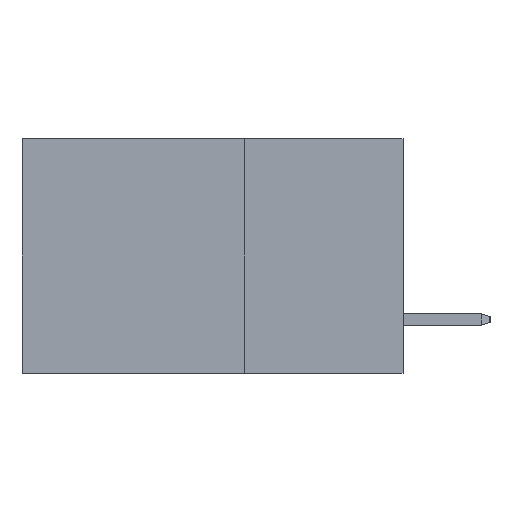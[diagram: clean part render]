
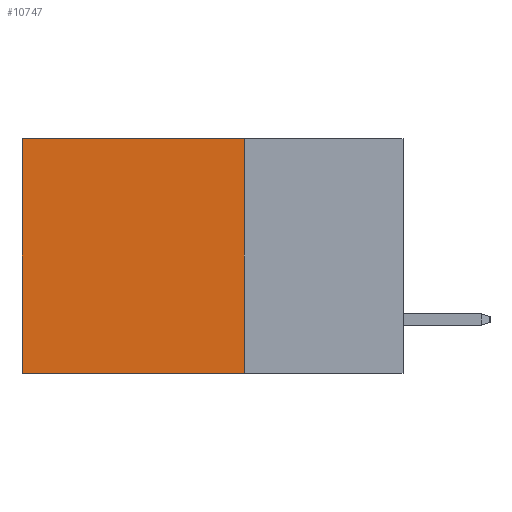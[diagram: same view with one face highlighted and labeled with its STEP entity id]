
A CAD part, left-side view. The second image highlights one B-rep face of the part: STEP entity #10747.
In plain terms, the highlighted planar face has unit normal (-1, 0, 0).
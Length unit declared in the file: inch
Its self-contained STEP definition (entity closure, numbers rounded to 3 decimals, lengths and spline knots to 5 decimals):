
#236 = ORIENTED_EDGE ( 'NONE', *, *, #14574, .T. ) ;
#462 = CARTESIAN_POINT ( 'NONE',  ( 0.2875, 0.25, 0. ) ) ;
#2843 = DIRECTION ( 'NONE',  ( 0., 1., 0. ) ) ;
#3055 = CARTESIAN_POINT ( 'NONE',  ( 0.2875, 0.6, -0.37 ) ) ;
#3961 = CARTESIAN_POINT ( 'NONE',  ( 0.2875, 0.25, 0. ) ) ;
#4391 = DIRECTION ( 'NONE',  ( 0., 0., -1. ) ) ;
#4435 = ORIENTED_EDGE ( 'NONE', *, *, #14207, .T. ) ;
#4590 = DIRECTION ( 'NONE',  ( 0., 1., 0. ) ) ;
#6143 = CARTESIAN_POINT ( 'NONE',  ( 0.2875, 0.25, -0.37 ) ) ;
#6612 = LINE ( 'NONE', #13173, #8025 ) ;
#6643 = VERTEX_POINT ( 'NONE', #3961 ) ;
#7412 = LINE ( 'NONE', #6143, #10661 ) ;
#7581 = VERTEX_POINT ( 'NONE', #9153 ) ;
#7586 = VERTEX_POINT ( 'NONE', #3055 ) ;
#8025 = VECTOR ( 'NONE', #4391, 39.37008 ) ;
#9153 = CARTESIAN_POINT ( 'NONE',  ( 0.2875, 0.6, 0. ) ) ;
#9303 = CARTESIAN_POINT ( 'NONE',  ( 0.2875, 0.25, 0. ) ) ;
#10048 = CARTESIAN_POINT ( 'NONE',  ( 0.2875, 0.25, -0.37 ) ) ;
#10375 = LINE ( 'NONE', #15325, #14056 ) ;
#10478 = PLANE ( 'NONE',  #12151 ) ;
#10661 = VECTOR ( 'NONE', #4590, 39.37008 ) ;
#10747 = ADVANCED_FACE ( 'NONE', ( #11766 ), #10478, .F. ) ;
#11629 = LINE ( 'NONE', #462, #13555 ) ;
#11670 = ORIENTED_EDGE ( 'NONE', *, *, #13518, .F. ) ;
#11766 = FACE_OUTER_BOUND ( 'NONE', #14147, .T. ) ;
#11843 = DIRECTION ( 'NONE',  ( 1., 0., 0. ) ) ;
#12151 = AXIS2_PLACEMENT_3D ( 'NONE', #9303, #11843, #14352 ) ;
#12481 = DIRECTION ( 'NONE',  ( 0., 0., -1. ) ) ;
#13173 = CARTESIAN_POINT ( 'NONE',  ( 0.2875, 0.6, 0. ) ) ;
#13518 = EDGE_CURVE ( 'NONE', #14947, #7586, #7412, .T. ) ;
#13555 = VECTOR ( 'NONE', #2843, 39.37008 ) ;
#13699 = EDGE_CURVE ( 'NONE', #6643, #14947, #10375, .T. ) ;
#14056 = VECTOR ( 'NONE', #12481, 39.37008 ) ;
#14147 = EDGE_LOOP ( 'NONE', ( #4435, #11670, #14569, #236 ) ) ;
#14207 = EDGE_CURVE ( 'NONE', #7581, #7586, #6612, .T. ) ;
#14352 = DIRECTION ( 'NONE',  ( 0., 0., -1. ) ) ;
#14569 = ORIENTED_EDGE ( 'NONE', *, *, #13699, .F. ) ;
#14574 = EDGE_CURVE ( 'NONE', #6643, #7581, #11629, .T. ) ;
#14947 = VERTEX_POINT ( 'NONE', #10048 ) ;
#15325 = CARTESIAN_POINT ( 'NONE',  ( 0.2875, 0.25, 0. ) ) ;
